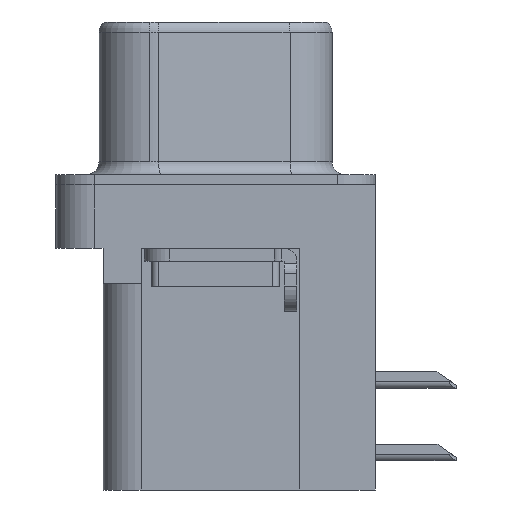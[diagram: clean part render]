
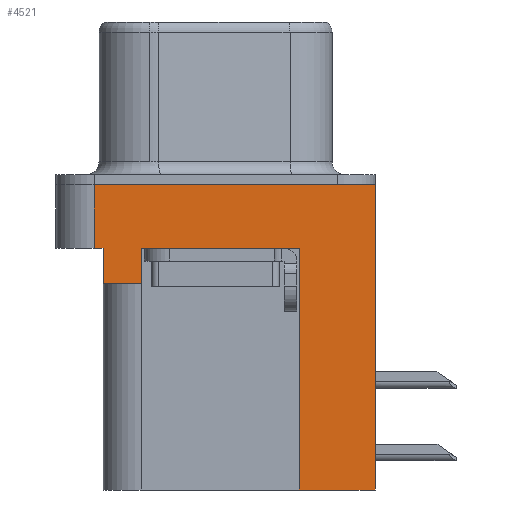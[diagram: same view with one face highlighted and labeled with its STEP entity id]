
A CAD part, left-side view. The second image highlights one B-rep face of the part: STEP entity #4521.
In plain terms, the highlighted planar face has unit normal (-1, 0, 0).
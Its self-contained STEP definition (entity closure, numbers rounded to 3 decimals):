
#332 = VERTEX_POINT ( 'NONE', #3372 ) ;
#405 = VERTEX_POINT ( 'NONE', #16908 ) ;
#526 = CARTESIAN_POINT ( 'NONE',  ( -2.935, -6.275, -2.5 ) ) ;
#669 = VERTEX_POINT ( 'NONE', #16164 ) ;
#1794 = EDGE_CURVE ( 'NONE', #3118, #17273, #5105, .T. ) ;
#2125 = CARTESIAN_POINT ( 'NONE',  ( -2.935, -6.275, -2.5 ) ) ;
#2132 = CARTESIAN_POINT ( 'NONE',  ( -2.935, 4.775, 0. ) ) ;
#2258 = EDGE_CURVE ( 'NONE', #332, #15633, #3081, .T. ) ;
#2774 = CARTESIAN_POINT ( 'NONE',  ( -2.935, 2.895, -2.5 ) ) ;
#2943 = VECTOR ( 'NONE', #13489, 1000. ) ;
#3081 = LINE ( 'NONE', #526, #2943 ) ;
#3118 = VERTEX_POINT ( 'NONE', #5118 ) ;
#3181 = CARTESIAN_POINT ( 'NONE',  ( -2.935, -3.295, -12. ) ) ;
#3372 = CARTESIAN_POINT ( 'NONE',  ( -2.935, 4.775, -2.5 ) ) ;
#3467 = ORIENTED_EDGE ( 'NONE', *, *, #4003, .F. ) ;
#3944 = VERTEX_POINT ( 'NONE', #14157 ) ;
#4003 = EDGE_CURVE ( 'NONE', #6899, #5235, #10897, .T. ) ;
#4090 = ORIENTED_EDGE ( 'NONE', *, *, #1794, .F. ) ;
#4125 = VECTOR ( 'NONE', #7432, 1000. ) ;
#4311 = LINE ( 'NONE', #5896, #4125 ) ;
#4328 = EDGE_CURVE ( 'NONE', #332, #6899, #8523, .T. ) ;
#4342 = VECTOR ( 'NONE', #7894, 1000. ) ;
#4488 = VECTOR ( 'NONE', #8496, 1000. ) ;
#4521 = ADVANCED_FACE ( 'NONE', ( #8084 ), #6457, .T. ) ;
#4581 = LINE ( 'NONE', #10942, #4488 ) ;
#4730 = LINE ( 'NONE', #8948, #4342 ) ;
#4754 = EDGE_CURVE ( 'NONE', #17273, #15633, #7571, .T. ) ;
#4984 = VECTOR ( 'NONE', #17426, 1000. ) ;
#5105 = LINE ( 'NONE', #15248, #4984 ) ;
#5118 = CARTESIAN_POINT ( 'NONE',  ( -2.935, 2.895, -3.9 ) ) ;
#5148 = EDGE_CURVE ( 'NONE', #3944, #669, #5562, .T. ) ;
#5163 = VECTOR ( 'NONE', #6546, 1000. ) ;
#5235 = VERTEX_POINT ( 'NONE', #8037 ) ;
#5281 = EDGE_CURVE ( 'NONE', #405, #3944, #4581, .T. ) ;
#5304 = EDGE_CURVE ( 'NONE', #405, #5235, #4730, .T. ) ;
#5562 = LINE ( 'NONE', #3181, #5163 ) ;
#5896 = CARTESIAN_POINT ( 'NONE',  ( -2.935, 2.895, -3.9 ) ) ;
#6299 = DIRECTION ( 'NONE',  ( 0., -1., 0. ) ) ;
#6369 = EDGE_CURVE ( 'NONE', #10619, #669, #16518, .T. ) ;
#6416 = DIRECTION ( 'NONE',  ( 0., 0., 1. ) ) ;
#6457 = PLANE ( 'NONE',  #7651 ) ;
#6546 = DIRECTION ( 'NONE',  ( 0., 0., 1. ) ) ;
#6899 = VERTEX_POINT ( 'NONE', #2132 ) ;
#7411 = VECTOR ( 'NONE', #11181, 1000. ) ;
#7432 = DIRECTION ( 'NONE',  ( 0., 0., 1. ) ) ;
#7571 = LINE ( 'NONE', #11518, #7411 ) ;
#7651 = AXIS2_PLACEMENT_3D ( 'NONE', #2125, #13574, #6416 ) ;
#7706 = EDGE_LOOP ( 'NONE', ( #3467, #15950, #11189, #9667, #4090, #12642, #17970, #13831, #14965, #13183 ) ) ;
#7894 = DIRECTION ( 'NONE',  ( 0., 0., 1. ) ) ;
#8037 = CARTESIAN_POINT ( 'NONE',  ( -2.935, -6.275, 0. ) ) ;
#8084 = FACE_OUTER_BOUND ( 'NONE', #7706, .T. ) ;
#8154 = CARTESIAN_POINT ( 'NONE',  ( -2.935, 4.425, -2.5 ) ) ;
#8496 = DIRECTION ( 'NONE',  ( 0., 1., 0. ) ) ;
#8523 = LINE ( 'NONE', #18532, #8540 ) ;
#8540 = VECTOR ( 'NONE', #17322, 1000. ) ;
#8948 = CARTESIAN_POINT ( 'NONE',  ( -2.935, -6.275, -2.5 ) ) ;
#9667 = ORIENTED_EDGE ( 'NONE', *, *, #4754, .F. ) ;
#9972 = EDGE_CURVE ( 'NONE', #3118, #10619, #4311, .T. ) ;
#10510 = DIRECTION ( 'NONE',  ( 0., -1., 0. ) ) ;
#10619 = VERTEX_POINT ( 'NONE', #2774 ) ;
#10854 = VECTOR ( 'NONE', #6299, 1000. ) ;
#10897 = LINE ( 'NONE', #15108, #10854 ) ;
#10942 = CARTESIAN_POINT ( 'NONE',  ( -2.935, -3.295, -12. ) ) ;
#11181 = DIRECTION ( 'NONE',  ( 0., 0., 1. ) ) ;
#11189 = ORIENTED_EDGE ( 'NONE', *, *, #2258, .T. ) ;
#11518 = CARTESIAN_POINT ( 'NONE',  ( -2.935, 4.425, -3.9 ) ) ;
#12642 = ORIENTED_EDGE ( 'NONE', *, *, #9972, .T. ) ;
#13183 = ORIENTED_EDGE ( 'NONE', *, *, #5304, .T. ) ;
#13489 = DIRECTION ( 'NONE',  ( 0., -1., 0. ) ) ;
#13574 = DIRECTION ( 'NONE',  ( -1., 0., 0. ) ) ;
#13831 = ORIENTED_EDGE ( 'NONE', *, *, #5148, .F. ) ;
#14157 = CARTESIAN_POINT ( 'NONE',  ( -2.935, -3.295, -12. ) ) ;
#14653 = CARTESIAN_POINT ( 'NONE',  ( -2.935, 4.425, -3.9 ) ) ;
#14965 = ORIENTED_EDGE ( 'NONE', *, *, #5281, .F. ) ;
#15108 = CARTESIAN_POINT ( 'NONE',  ( -2.935, -6.275, 0. ) ) ;
#15248 = CARTESIAN_POINT ( 'NONE',  ( -2.935, 4.425, -3.9 ) ) ;
#15633 = VERTEX_POINT ( 'NONE', #8154 ) ;
#15872 = CARTESIAN_POINT ( 'NONE',  ( -2.935, -6.275, -2.5 ) ) ;
#15950 = ORIENTED_EDGE ( 'NONE', *, *, #4328, .F. ) ;
#16164 = CARTESIAN_POINT ( 'NONE',  ( -2.935, -3.295, -2.5 ) ) ;
#16505 = VECTOR ( 'NONE', #10510, 1000. ) ;
#16518 = LINE ( 'NONE', #15872, #16505 ) ;
#16908 = CARTESIAN_POINT ( 'NONE',  ( -2.935, -6.275, -12. ) ) ;
#17273 = VERTEX_POINT ( 'NONE', #14653 ) ;
#17322 = DIRECTION ( 'NONE',  ( 0., 0., 1. ) ) ;
#17426 = DIRECTION ( 'NONE',  ( 0., 1., 0. ) ) ;
#17970 = ORIENTED_EDGE ( 'NONE', *, *, #6369, .T. ) ;
#18532 = CARTESIAN_POINT ( 'NONE',  ( -2.935, 4.775, -2.5 ) ) ;
